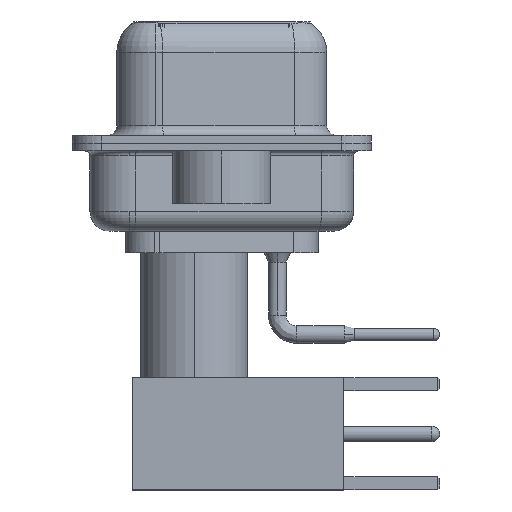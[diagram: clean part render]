
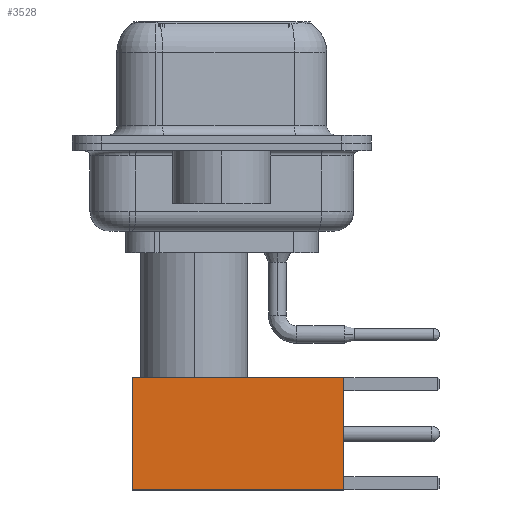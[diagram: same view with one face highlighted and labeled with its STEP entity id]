
A CAD part, left-side view. The second image highlights one B-rep face of the part: STEP entity #3528.
In plain terms, the highlighted face is planar.
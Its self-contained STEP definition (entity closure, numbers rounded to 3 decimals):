
#924 = ORIENTED_EDGE ( 'NONE', *, *, #22435, .T. ) ;
#998 = EDGE_CURVE ( 'NONE', #9215, #1958, #14643, .T. ) ;
#1958 = VERTEX_POINT ( 'NONE', #25460 ) ;
#2352 = ORIENTED_EDGE ( 'NONE', *, *, #4055, .T. ) ;
#2524 = CARTESIAN_POINT ( 'NONE',  ( 0., 2.875, 10.82 ) ) ;
#3078 = CARTESIAN_POINT ( 'NONE',  ( 2.875, 2.875, 0. ) ) ;
#3173 = VECTOR ( 'NONE', #6898, 1000. ) ;
#3528 = ADVANCED_FACE ( 'NONE', ( #19012 ), #21117, .T. ) ;
#4055 = EDGE_CURVE ( 'NONE', #9555, #20779, #23449, .T. ) ;
#6603 = EDGE_CURVE ( 'NONE', #1958, #20779, #16548, .T. ) ;
#6898 = DIRECTION ( 'NONE',  ( 0., 0., -1. ) ) ;
#8580 = CARTESIAN_POINT ( 'NONE',  ( 2.875, 2.875, 0. ) ) ;
#9215 = VERTEX_POINT ( 'NONE', #12788 ) ;
#9351 = CARTESIAN_POINT ( 'NONE',  ( 0., 2.875, 0. ) ) ;
#9555 = VERTEX_POINT ( 'NONE', #23977 ) ;
#10250 = VECTOR ( 'NONE', #20957, 1000. ) ;
#12591 = VECTOR ( 'NONE', #18592, 1000. ) ;
#12788 = CARTESIAN_POINT ( 'NONE',  ( 2.875, 2.875, 10.82 ) ) ;
#12964 = DIRECTION ( 'NONE',  ( 0., 1., 0. ) ) ;
#14643 = LINE ( 'NONE', #2524, #12591 ) ;
#14746 = CARTESIAN_POINT ( 'NONE',  ( -2.875, 2.875, 0. ) ) ;
#15027 = LINE ( 'NONE', #8580, #10250 ) ;
#15299 = DIRECTION ( 'NONE',  ( -1., 0., 0. ) ) ;
#15329 = DIRECTION ( 'NONE',  ( 0., 0., 1. ) ) ;
#16548 = LINE ( 'NONE', #24702, #3173 ) ;
#17707 = AXIS2_PLACEMENT_3D ( 'NONE', #3078, #12964, #15329 ) ;
#18592 = DIRECTION ( 'NONE',  ( -1., 0., 0. ) ) ;
#19012 = FACE_OUTER_BOUND ( 'NONE', #22345, .T. ) ;
#20779 = VERTEX_POINT ( 'NONE', #14746 ) ;
#20957 = DIRECTION ( 'NONE',  ( 0., 0., -1. ) ) ;
#20978 = VECTOR ( 'NONE', #15299, 1000. ) ;
#21117 = PLANE ( 'NONE',  #17707 ) ;
#21283 = ORIENTED_EDGE ( 'NONE', *, *, #6603, .F. ) ;
#22345 = EDGE_LOOP ( 'NONE', ( #924, #2352, #21283, #24482 ) ) ;
#22435 = EDGE_CURVE ( 'NONE', #9215, #9555, #15027, .T. ) ;
#23449 = LINE ( 'NONE', #9351, #20978 ) ;
#23977 = CARTESIAN_POINT ( 'NONE',  ( 2.875, 2.875, 0. ) ) ;
#24482 = ORIENTED_EDGE ( 'NONE', *, *, #998, .F. ) ;
#24702 = CARTESIAN_POINT ( 'NONE',  ( -2.875, 2.875, 0. ) ) ;
#25460 = CARTESIAN_POINT ( 'NONE',  ( -2.875, 2.875, 10.82 ) ) ;
